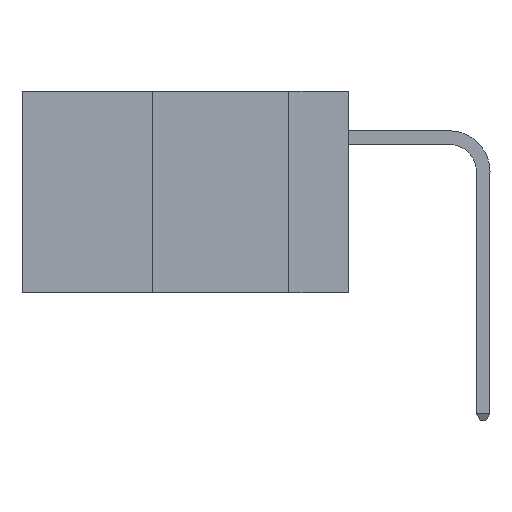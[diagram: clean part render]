
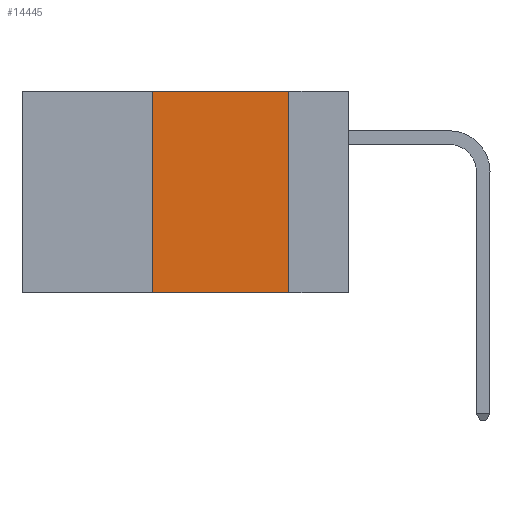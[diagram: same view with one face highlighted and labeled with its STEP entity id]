
A CAD part, left-side view. The second image highlights one B-rep face of the part: STEP entity #14445.
In plain terms, the highlighted planar face has unit normal (-1, 0, 0).
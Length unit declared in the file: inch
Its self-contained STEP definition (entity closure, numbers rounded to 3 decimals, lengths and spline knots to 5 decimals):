
#6 = PLANE ( 'NONE',  #8205 ) ;
#165 = CARTESIAN_POINT ( 'NONE',  ( 0., 0.11, 0. ) ) ;
#344 = VECTOR ( 'NONE', #10753, 39.37008 ) ;
#870 = LINE ( 'NONE', #16688, #344 ) ;
#1198 = EDGE_LOOP ( 'NONE', ( #12293, #12045, #5407, #7067 ) ) ;
#1688 = CARTESIAN_POINT ( 'NONE',  ( 0., 0.6, 0. ) ) ;
#1841 = DIRECTION ( 'NONE',  ( 0., -1., 0. ) ) ;
#1960 = LINE ( 'NONE', #13166, #10304 ) ;
#2259 = LINE ( 'NONE', #5033, #6811 ) ;
#3505 = EDGE_CURVE ( 'NONE', #12610, #5633, #2259, .T. ) ;
#3793 = VECTOR ( 'NONE', #4687, 39.37008 ) ;
#4181 = FACE_OUTER_BOUND ( 'NONE', #1198, .T. ) ;
#4687 = DIRECTION ( 'NONE',  ( 0., -1., 0. ) ) ;
#4735 = EDGE_CURVE ( 'NONE', #12767, #20214, #870, .T. ) ;
#5033 = CARTESIAN_POINT ( 'NONE',  ( 0., 0.36, 0. ) ) ;
#5167 = DIRECTION ( 'NONE',  ( 0., 0., -1. ) ) ;
#5407 = ORIENTED_EDGE ( 'NONE', *, *, #3505, .F. ) ;
#5633 = VERTEX_POINT ( 'NONE', #19185 ) ;
#6811 = VECTOR ( 'NONE', #20496, 39.37008 ) ;
#7067 = ORIENTED_EDGE ( 'NONE', *, *, #8562, .T. ) ;
#8205 = AXIS2_PLACEMENT_3D ( 'NONE', #1688, #14619, #5167 ) ;
#8562 = EDGE_CURVE ( 'NONE', #12610, #20214, #1960, .T. ) ;
#10304 = VECTOR ( 'NONE', #1841, 39.37008 ) ;
#10753 = DIRECTION ( 'NONE',  ( 0., 0., -1. ) ) ;
#12045 = ORIENTED_EDGE ( 'NONE', *, *, #17367, .F. ) ;
#12293 = ORIENTED_EDGE ( 'NONE', *, *, #4735, .F. ) ;
#12610 = VERTEX_POINT ( 'NONE', #20506 ) ;
#12767 = VERTEX_POINT ( 'NONE', #165 ) ;
#13166 = CARTESIAN_POINT ( 'NONE',  ( 0., 0.6, -0.37 ) ) ;
#14181 = CARTESIAN_POINT ( 'NONE',  ( 0., 0.6, 0. ) ) ;
#14445 = ADVANCED_FACE ( 'NONE', ( #4181 ), #6, .F. ) ;
#14619 = DIRECTION ( 'NONE',  ( 1., 0., 0. ) ) ;
#16688 = CARTESIAN_POINT ( 'NONE',  ( 0., 0.11, 0. ) ) ;
#17367 = EDGE_CURVE ( 'NONE', #5633, #12767, #20556, .T. ) ;
#19127 = CARTESIAN_POINT ( 'NONE',  ( 0., 0.11, -0.37 ) ) ;
#19185 = CARTESIAN_POINT ( 'NONE',  ( 0., 0.36, 0. ) ) ;
#20214 = VERTEX_POINT ( 'NONE', #19127 ) ;
#20496 = DIRECTION ( 'NONE',  ( 0., 0., 1. ) ) ;
#20506 = CARTESIAN_POINT ( 'NONE',  ( 0., 0.36, -0.37 ) ) ;
#20556 = LINE ( 'NONE', #14181, #3793 ) ;
